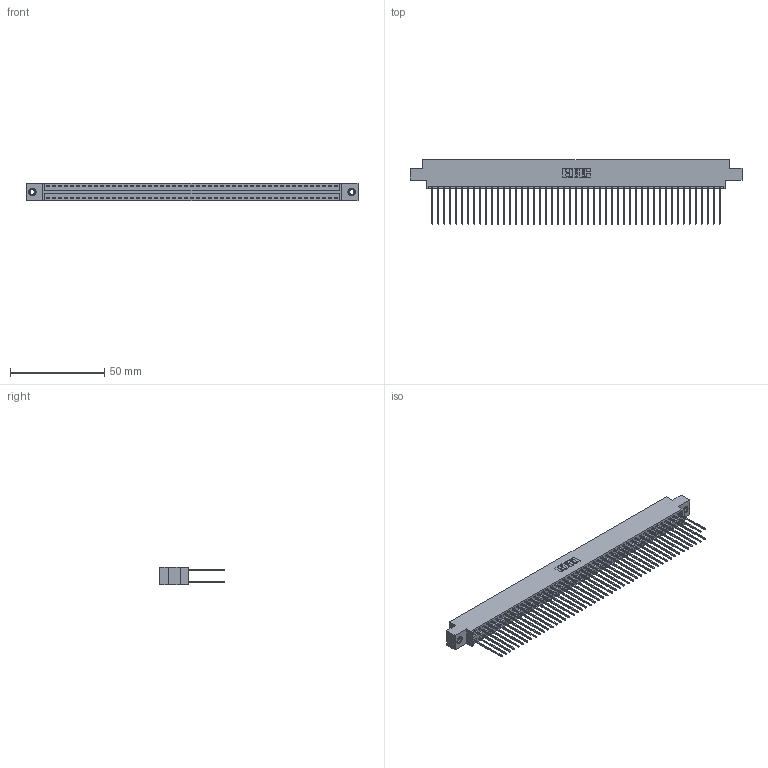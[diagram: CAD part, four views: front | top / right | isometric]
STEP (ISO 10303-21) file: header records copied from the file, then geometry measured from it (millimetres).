
FILE_DESCRIPTION (( 'STEP AP203' ), '1' );
FILE_NAME ('346-098-541-807.STEP', '2022-05-26T18:37:22', ( '' ), ( '' ), 'SwSTEP 2.0', 'SolidWorks 2020', '' );
FILE_SCHEMA (( 'CONFIG_CONTROL_DESIGN' ));
Length unit declared in the file: inch
Products named in the file (4): 346-098-541-807; 345-292-001_345-293-141; 345-250-001_345-250-005-103; 346 Part_0.170 Offset - 0.156 Dia-TI
Assembly tree (101 placements, depth 2):
  346-098-541-807
    346 Part_0.170 Offset - 0.156 Dia-TI
    345-292-001_345-293-141  x98
    345-250-001_345-250-005-103  x2
Bounding box: 176.15 x 34.29 x 9.4 mm (x, y, z)
Volume: 17625.2 mm3; surface area: 27246.8 mm2
Topology: 101 solids, 101 shells, 5282 faces, 15667 edges, 10306 vertices
Faces by surface type: plane 3542, cylinder 1724, cone 12, torus 4
Entity records: 32372 total; most frequent: CARTESIAN_POINT 5311, ORIENTED_EDGE 5238, DIRECTION 4757, EDGE_CURVE 2619, LINE 2271, VECTOR 2271, VERTEX_POINT 1740, AXIS2_PLACEMENT_3D 1243
